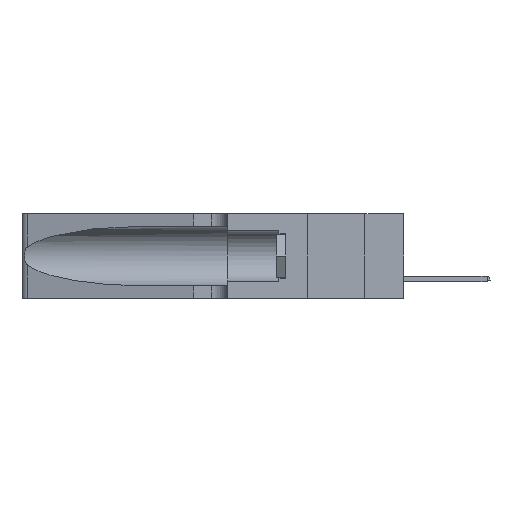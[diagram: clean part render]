
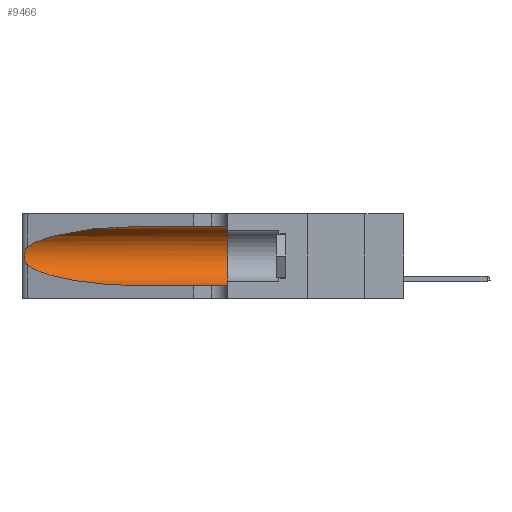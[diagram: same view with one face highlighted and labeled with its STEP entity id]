
A CAD part, left-side view. The second image highlights one B-rep face of the part: STEP entity #9466.
In plain terms, the highlighted cylindrical face has radius 3.308 mm (diameter 6.617 mm), a partial arc.
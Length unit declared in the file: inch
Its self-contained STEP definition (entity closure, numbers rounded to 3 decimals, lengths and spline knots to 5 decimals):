
#422 = DIRECTION ( 'NONE',  ( 0., 0., -1. ) ) ;
#860 = CARTESIAN_POINT ( 'NONE',  ( 0.1305, 0.35, 0.31525 ) ) ;
#892 = CIRCLE ( 'NONE', #27359, 0.13025 ) ;
#1110 = CARTESIAN_POINT ( 'NONE',  ( 0.25487, 1.22718, 0.14631 ) ) ;
#2375 = ORIENTED_EDGE ( 'NONE', *, *, #12904, .F. ) ;
#2853 = CARTESIAN_POINT ( 'NONE',  ( 0.25487, 1.22718, 0.14631 ) ) ;
#2962 = CARTESIAN_POINT ( 'NONE',  ( 0.25555, 1.22993, 0.14849 ) ) ;
#3661 = CARTESIAN_POINT ( 'NONE',  ( 0.25639, 1.23184, 0.21858 ) ) ;
#4594 = ORIENTED_EDGE ( 'NONE', *, *, #7871, .T. ) ;
#4603 = CYLINDRICAL_SURFACE ( 'NONE', #29641, 0.13025 ) ;
#4669 = CARTESIAN_POINT ( 'NONE',  ( 0.26018, 1.23835, 0.19895 ) ) ;
#5050 = VERTEX_POINT ( 'NONE', #860 ) ;
#5448 = FACE_OUTER_BOUND ( 'NONE', #22977, .T. ) ;
#7087 = DIRECTION ( 'NONE',  ( 0., -1., 0. ) ) ;
#7871 = EDGE_CURVE ( 'NONE', #21205, #10678, #10741, .T. ) ;
#8109 = VERTEX_POINT ( 'NONE', #15750 ) ;
#8409 = VECTOR ( 'NONE', #30868, 39.37008 ) ;
#8915 = EDGE_CURVE ( 'NONE', #28614, #8109, #22881, .T. ) ;
#9466 = ADVANCED_FACE ( 'NONE', ( #5448 ), #4603, .F. ) ;
#10201 = EDGE_CURVE ( 'NONE', #10678, #28614, #30757, .T. ) ;
#10475 = CARTESIAN_POINT ( 'NONE',  ( 0.1305, 1.61858, 0.31525 ) ) ;
#10678 = VERTEX_POINT ( 'NONE', #1110 ) ;
#10741 = B_SPLINE_CURVE_WITH_KNOTS ( 'NONE', 3,
 ( #13184, #34743, #3661, #31317, #17797, #4669, #10975, #19656, #22400, #27920, #32835, #35131, #2962, #2853 ),
 .UNSPECIFIED., .F., .F.,
 ( 4, 2, 2, 2, 2, 2, 4 ),
 ( 0., 0.00027, 0.00053, 0.00107, 0.0016, 0.00187, 0.00214 ),
 .UNSPECIFIED. ) ;
#10975 = CARTESIAN_POINT ( 'NONE',  ( 0.26075, 1.23896, 0.19203 ) ) ;
#12277 = CARTESIAN_POINT ( 'NONE',  ( 0.25487, 1.22718, 0.22369 ) ) ;
#12904 = EDGE_CURVE ( 'NONE', #22241, #5050, #28685, .T. ) ;
#13184 = CARTESIAN_POINT ( 'NONE',  ( 0.25487, 1.22718, 0.22369 ) ) ;
#14548 = DIRECTION ( 'NONE',  ( 0., 1., 0. ) ) ;
#15750 = CARTESIAN_POINT ( 'NONE',  ( 0.1305, 0.35, 0.05475 ) ) ;
#15941 = DIRECTION ( 'NONE',  ( 0., -1., 0. ) ) ;
#16888 = CARTESIAN_POINT ( 'NONE',  ( 0.1305, 0.35, 0.185 ) ) ;
#17532 = ORIENTED_EDGE ( 'NONE', *, *, #10201, .T. ) ;
#17797 = CARTESIAN_POINT ( 'NONE',  ( 0.25854, 1.2359, 0.20912 ) ) ;
#17964 = CARTESIAN_POINT ( 'NONE',  ( 0.2373, 1.15595, 0.28018 ) ) ;
#19635 = DIRECTION ( 'NONE',  ( 0., 0., 1. ) ) ;
#19656 = CARTESIAN_POINT ( 'NONE',  ( 0.26075, 1.23896, 0.178 ) ) ;
#19961 = CARTESIAN_POINT ( 'NONE',  ( 0.1305, 0.72297, 0.05475 ) ) ;
#20327 = CARTESIAN_POINT ( 'NONE',  ( 0.25487, 1.22718, 0.14631 ) ) ;
#20788 =( BOUNDED_CURVE ( )  B_SPLINE_CURVE ( 3, ( #34097, #34216, #17964, #12277 ),
 .UNSPECIFIED., .F., .F. ) 
 B_SPLINE_CURVE_WITH_KNOTS ( ( 4, 4 ),
 ( 1.5708, 2.84003 ),
 .UNSPECIFIED. ) 
 CURVE ( )  GEOMETRIC_REPRESENTATION_ITEM ( )  RATIONAL_B_SPLINE_CURVE ( ( 1., 0.87, 0.87, 1. ) ) 
 REPRESENTATION_ITEM ( '' )  );
#21205 = VERTEX_POINT ( 'NONE', #22928 ) ;
#22241 = VERTEX_POINT ( 'NONE', #33563 ) ;
#22400 = CARTESIAN_POINT ( 'NONE',  ( 0.26017, 1.23833, 0.17102 ) ) ;
#22881 = LINE ( 'NONE', #28166, #8409 ) ;
#22928 = CARTESIAN_POINT ( 'NONE',  ( 0.25487, 1.22718, 0.22369 ) ) ;
#22936 = CARTESIAN_POINT ( 'NONE',  ( 0.2373, 1.15595, 0.08982 ) ) ;
#22977 = EDGE_LOOP ( 'NONE', ( #29745, #4594, #17532, #33176, #23875, #2375 ) ) ;
#23705 = CARTESIAN_POINT ( 'NONE',  ( 0.1305, 1.61858, 0.185 ) ) ;
#23875 = ORIENTED_EDGE ( 'NONE', *, *, #31528, .F. ) ;
#25344 = CARTESIAN_POINT ( 'NONE',  ( 0.1305, 0.72297, 0.05475 ) ) ;
#27359 = AXIS2_PLACEMENT_3D ( 'NONE', #16888, #14548, #19635 ) ;
#27551 = EDGE_CURVE ( 'NONE', #22241, #21205, #20788, .T. ) ;
#27920 = CARTESIAN_POINT ( 'NONE',  ( 0.25856, 1.23593, 0.16098 ) ) ;
#28166 = CARTESIAN_POINT ( 'NONE',  ( 0.1305, 1.61858, 0.05475 ) ) ;
#28614 = VERTEX_POINT ( 'NONE', #25344 ) ;
#28685 = LINE ( 'NONE', #10475, #31186 ) ;
#29641 = AXIS2_PLACEMENT_3D ( 'NONE', #23705, #7087, #422 ) ;
#29745 = ORIENTED_EDGE ( 'NONE', *, *, #27551, .T. ) ;
#30757 =( BOUNDED_CURVE ( )  B_SPLINE_CURVE ( 3, ( #20327, #22936, #30884, #19961 ),
 .UNSPECIFIED., .F., .F. ) 
 B_SPLINE_CURVE_WITH_KNOTS ( ( 4, 4 ),
 ( 3.44316, 4.71239 ),
 .UNSPECIFIED. ) 
 CURVE ( )  GEOMETRIC_REPRESENTATION_ITEM ( )  RATIONAL_B_SPLINE_CURVE ( ( 1., 0.87, 0.87, 1. ) ) 
 REPRESENTATION_ITEM ( '' )  );
#30868 = DIRECTION ( 'NONE',  ( 0., -1., 0. ) ) ;
#30884 = CARTESIAN_POINT ( 'NONE',  ( 0.18966, 0.96281, 0.05475 ) ) ;
#31186 = VECTOR ( 'NONE', #15941, 39.37008 ) ;
#31317 = CARTESIAN_POINT ( 'NONE',  ( 0.25787, 1.23484, 0.2124 ) ) ;
#31528 = EDGE_CURVE ( 'NONE', #5050, #8109, #892, .T. ) ;
#32835 = CARTESIAN_POINT ( 'NONE',  ( 0.25789, 1.23486, 0.15765 ) ) ;
#33176 = ORIENTED_EDGE ( 'NONE', *, *, #8915, .T. ) ;
#33563 = CARTESIAN_POINT ( 'NONE',  ( 0.1305, 0.72297, 0.31525 ) ) ;
#34097 = CARTESIAN_POINT ( 'NONE',  ( 0.1305, 0.72297, 0.31525 ) ) ;
#34216 = CARTESIAN_POINT ( 'NONE',  ( 0.18966, 0.96281, 0.31525 ) ) ;
#34743 = CARTESIAN_POINT ( 'NONE',  ( 0.25555, 1.22994, 0.2215 ) ) ;
#35131 = CARTESIAN_POINT ( 'NONE',  ( 0.25639, 1.23186, 0.15144 ) ) ;
